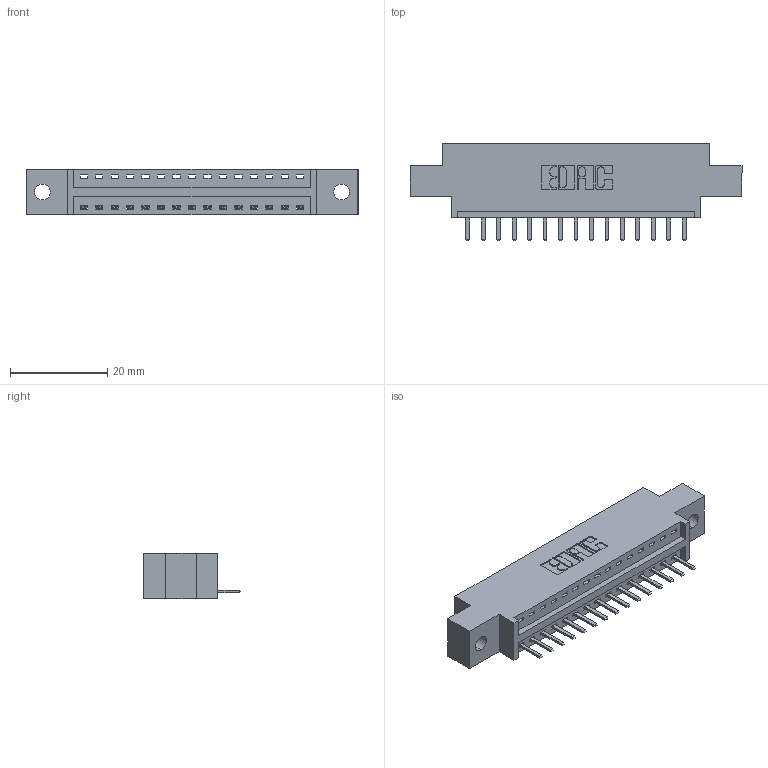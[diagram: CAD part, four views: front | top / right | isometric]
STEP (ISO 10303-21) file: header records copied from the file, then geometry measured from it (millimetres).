
FILE_DESCRIPTION (( 'STEP AP203' ), '1' );
FILE_NAME ('396-015-520-602.STEP', '2018-08-31T11:38:05', ( '' ), ( '' ), 'SwSTEP 2.0', 'SolidWorks 2016', '' );
FILE_SCHEMA (( 'CONFIG_CONTROL_DESIGN' ));
Length unit declared in the file: inch
Products named in the file (3): 346 Part_0.170 Offset - 0.128 Dia; 345-292-001_345-293-120; 396-015-520-602
Assembly tree (16 placements, depth 2):
  396-015-520-602
    346 Part_0.170 Offset - 0.128 Dia
    345-292-001_345-293-120  x15
Bounding box: 68.2 x 20.02 x 9.4 mm (x, y, z)
Volume: 6107.7 mm3; surface area: 7087.5 mm2
Topology: 16 solids, 16 shells, 1056 faces, 3101 edges, 2026 vertices
Faces by surface type: plane 710, cylinder 346
Entity records: 13193 total; most frequent: CARTESIAN_POINT 2289, ORIENTED_EDGE 2226, DIRECTION 2039, EDGE_CURVE 1113, VECTOR 917, LINE 917, VERTEX_POINT 738, AXIS2_PLACEMENT_3D 561
